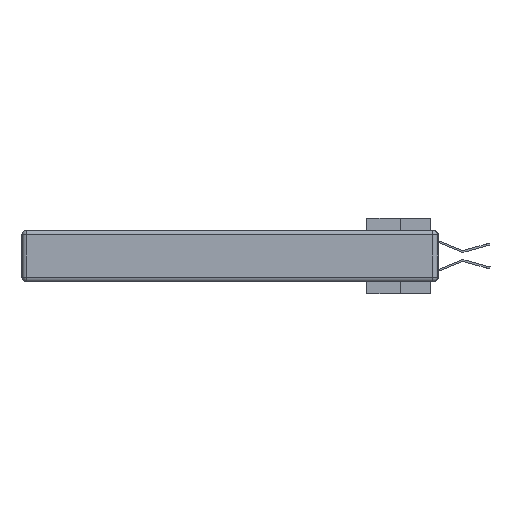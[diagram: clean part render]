
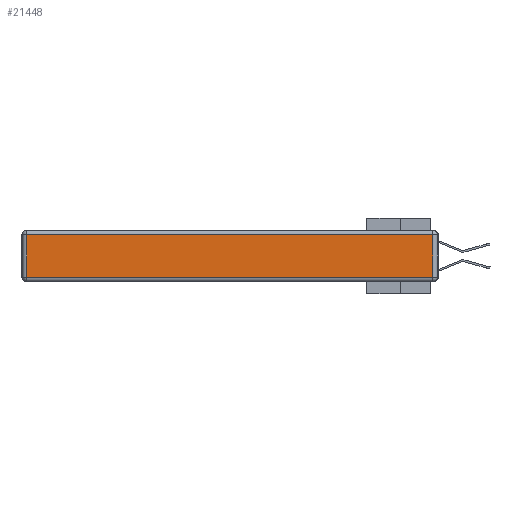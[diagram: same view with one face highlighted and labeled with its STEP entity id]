
A CAD part, left-side view. The second image highlights one B-rep face of the part: STEP entity #21448.
In plain terms, the highlighted planar face has unit normal (-1, 0, 0).
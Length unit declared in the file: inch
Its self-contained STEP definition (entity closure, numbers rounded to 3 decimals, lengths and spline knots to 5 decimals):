
#140 = CARTESIAN_POINT ( 'NONE',  ( 0., 2.72, -0.343 ) ) ;
#359 = VERTEX_POINT ( 'NONE', #19652 ) ;
#605 = EDGE_CURVE ( 'NONE', #13882, #18212, #23816, .T. ) ;
#1309 = LINE ( 'NONE', #140, #14709 ) ;
#8129 = ORIENTED_EDGE ( 'NONE', *, *, #605, .T. ) ;
#8788 = EDGE_CURVE ( 'NONE', #18212, #359, #12379, .T. ) ;
#9155 = DIRECTION ( 'NONE',  ( 0., 0., -1. ) ) ;
#9634 = PLANE ( 'NONE',  #34774 ) ;
#12266 = DIRECTION ( 'NONE',  ( 0., 1., 0. ) ) ;
#12379 = LINE ( 'NONE', #25493, #17233 ) ;
#13358 = ORIENTED_EDGE ( 'NONE', *, *, #8788, .T. ) ;
#13882 = VERTEX_POINT ( 'NONE', #39400 ) ;
#14709 = VECTOR ( 'NONE', #9155, 39.37008 ) ;
#15606 = VECTOR ( 'NONE', #24376, 39.37008 ) ;
#16087 = DIRECTION ( 'NONE',  ( -1., 0., 0. ) ) ;
#17233 = VECTOR ( 'NONE', #22427, 39.37008 ) ;
#18005 = LINE ( 'NONE', #37039, #33634 ) ;
#18212 = VERTEX_POINT ( 'NONE', #27658 ) ;
#18738 = ORIENTED_EDGE ( 'NONE', *, *, #28705, .T. ) ;
#19652 = CARTESIAN_POINT ( 'NONE',  ( 0., 0.03, -0.03 ) ) ;
#21448 = ADVANCED_FACE ( 'NONE', ( #27750 ), #9634, .T. ) ;
#22427 = DIRECTION ( 'NONE',  ( 0., 0., 1. ) ) ;
#23301 = CARTESIAN_POINT ( 'NONE',  ( 0., 2.72, -0.03 ) ) ;
#23816 = LINE ( 'NONE', #24498, #15606 ) ;
#24376 = DIRECTION ( 'NONE',  ( 0., -1., 0. ) ) ;
#24498 = CARTESIAN_POINT ( 'NONE',  ( 0., 0., -0.313 ) ) ;
#25493 = CARTESIAN_POINT ( 'NONE',  ( 0., 0.03, -0.343 ) ) ;
#27658 = CARTESIAN_POINT ( 'NONE',  ( 0., 0.03, -0.313 ) ) ;
#27750 = FACE_OUTER_BOUND ( 'NONE', #32484, .T. ) ;
#28391 = CARTESIAN_POINT ( 'NONE',  ( 0., 0., -0.343 ) ) ;
#28554 = VERTEX_POINT ( 'NONE', #23301 ) ;
#28705 = EDGE_CURVE ( 'NONE', #28554, #13882, #1309, .T. ) ;
#29878 = EDGE_CURVE ( 'NONE', #359, #28554, #18005, .T. ) ;
#31148 = DIRECTION ( 'NONE',  ( 0., 0., 1. ) ) ;
#32484 = EDGE_LOOP ( 'NONE', ( #8129, #13358, #34843, #18738 ) ) ;
#33634 = VECTOR ( 'NONE', #12266, 39.37008 ) ;
#34774 = AXIS2_PLACEMENT_3D ( 'NONE', #28391, #16087, #31148 ) ;
#34843 = ORIENTED_EDGE ( 'NONE', *, *, #29878, .T. ) ;
#37039 = CARTESIAN_POINT ( 'NONE',  ( 0., 2.75, -0.03 ) ) ;
#39400 = CARTESIAN_POINT ( 'NONE',  ( 0., 2.72, -0.313 ) ) ;
